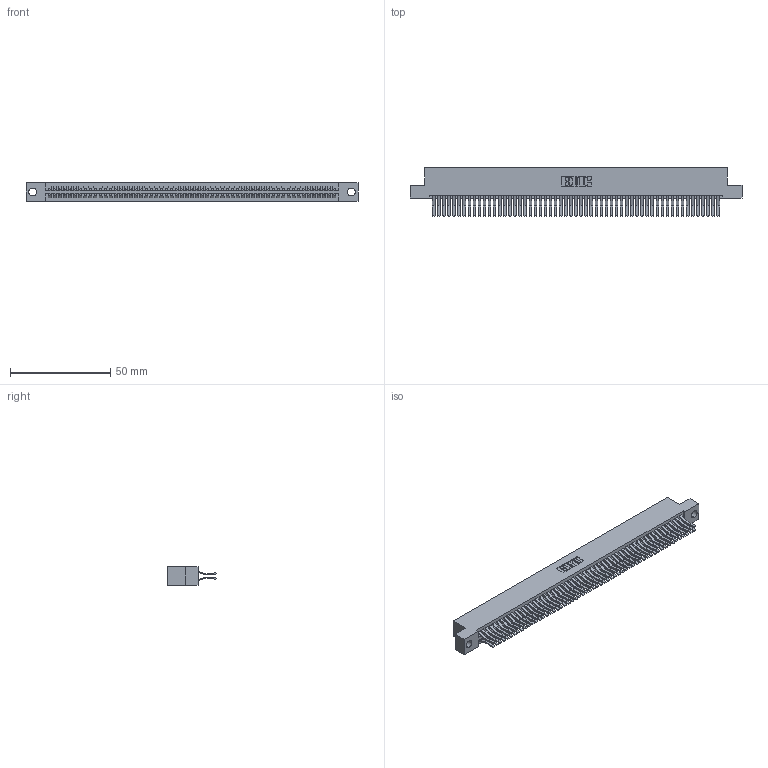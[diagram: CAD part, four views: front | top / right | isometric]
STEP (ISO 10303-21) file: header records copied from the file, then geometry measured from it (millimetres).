
FILE_DESCRIPTION (( 'STEP AP203' ), '1' );
FILE_NAME ('395-114-560-204.STEP', '2021-06-17T19:11:56', ( '' ), ( '' ), 'SwSTEP 2.0', 'SolidWorks 2020', '' );
FILE_SCHEMA (( 'CONFIG_CONTROL_DESIGN' ));
Length unit declared in the file: inch
Products named in the file (3): 345 Part_Flush Mounting Lugs - 0.156 Dia-TI; 345-292-001_560 Tail; 395-114-560-204
Assembly tree (115 placements, depth 2):
  395-114-560-204
    345 Part_Flush Mounting Lugs - 0.156 Dia-TI
    345-292-001_560 Tail  x114
Bounding box: 165.99 x 24.45 x 9.4 mm (x, y, z)
Volume: 16904.9 mm3; surface area: 27052.1 mm2
Topology: 115 solids, 115 shells, 6068 faces, 18047 edges, 11878 vertices
Faces by surface type: plane 3856, cylinder 2212
Entity records: 43211 total; most frequent: CARTESIAN_POINT 7234, ORIENTED_EDGE 7166, DIRECTION 6363, EDGE_CURVE 3583, VECTOR 3219, LINE 3219, VERTEX_POINT 2386, AXIS2_PLACEMENT_3D 1572
